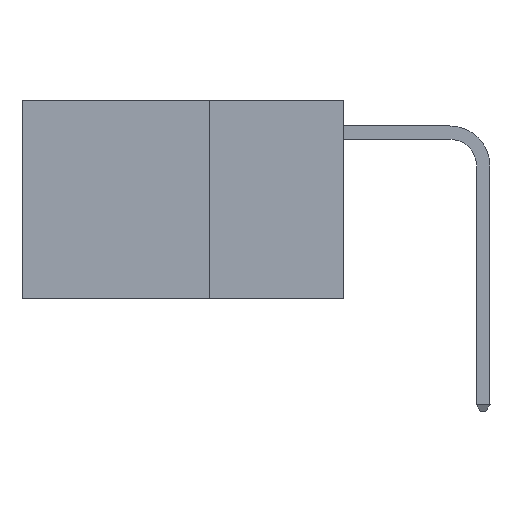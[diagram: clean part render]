
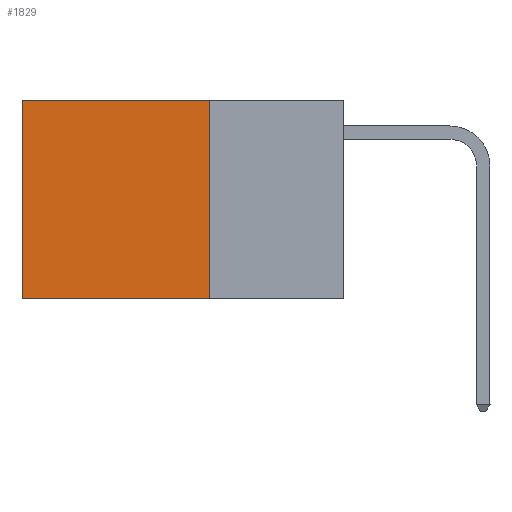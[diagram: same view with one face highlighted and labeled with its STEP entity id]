
A CAD part, left-side view. The second image highlights one B-rep face of the part: STEP entity #1829.
In plain terms, the highlighted planar face has unit normal (-1, 0, 0).
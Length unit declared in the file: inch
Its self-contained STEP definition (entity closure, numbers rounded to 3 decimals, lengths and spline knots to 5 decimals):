
#61 = EDGE_CURVE ( 'NONE', #5721, #1427, #5950, .T. ) ;
#127 = EDGE_CURVE ( 'NONE', #5721, #3329, #2680, .T. ) ;
#220 = PLANE ( 'NONE',  #3698 ) ;
#807 = CARTESIAN_POINT ( 'NONE',  ( 0.2625, 0.25, 0. ) ) ;
#833 = CARTESIAN_POINT ( 'NONE',  ( 0.2625, 0.25, 0. ) ) ;
#1358 = DIRECTION ( 'NONE',  ( 0., 0., -1. ) ) ;
#1413 = VECTOR ( 'NONE', #7861, 39.37008 ) ;
#1427 = VERTEX_POINT ( 'NONE', #7949 ) ;
#1829 = ADVANCED_FACE ( 'NONE', ( #3188 ), #220, .F. ) ;
#2013 = CARTESIAN_POINT ( 'NONE',  ( 0.2625, 0.25, -0.37 ) ) ;
#2420 = VECTOR ( 'NONE', #8285, 39.37008 ) ;
#2680 = LINE ( 'NONE', #5783, #2968 ) ;
#2968 = VECTOR ( 'NONE', #8905, 39.37008 ) ;
#3188 = FACE_OUTER_BOUND ( 'NONE', #7312, .T. ) ;
#3248 = DIRECTION ( 'NONE',  ( 1., 0., 0. ) ) ;
#3329 = VERTEX_POINT ( 'NONE', #4939 ) ;
#3698 = AXIS2_PLACEMENT_3D ( 'NONE', #807, #3248, #7219 ) ;
#3775 = EDGE_CURVE ( 'NONE', #1427, #8140, #5846, .T. ) ;
#4640 = CARTESIAN_POINT ( 'NONE',  ( 0.2625, 0.6, -0.37 ) ) ;
#4756 = VECTOR ( 'NONE', #1358, 39.37008 ) ;
#4757 = CARTESIAN_POINT ( 'NONE',  ( 0.2625, 0.6, 0. ) ) ;
#4939 = CARTESIAN_POINT ( 'NONE',  ( 0.2625, 0.6, 0. ) ) ;
#5721 = VERTEX_POINT ( 'NONE', #833 ) ;
#5783 = CARTESIAN_POINT ( 'NONE',  ( 0.2625, 0.25, 0. ) ) ;
#5846 = LINE ( 'NONE', #2013, #2420 ) ;
#5950 = LINE ( 'NONE', #9071, #4756 ) ;
#7047 = ORIENTED_EDGE ( 'NONE', *, *, #61, .F. ) ;
#7219 = DIRECTION ( 'NONE',  ( 0., 0., -1. ) ) ;
#7246 = ORIENTED_EDGE ( 'NONE', *, *, #3775, .F. ) ;
#7312 = EDGE_LOOP ( 'NONE', ( #7523, #7246, #7047, #9655 ) ) ;
#7523 = ORIENTED_EDGE ( 'NONE', *, *, #8175, .T. ) ;
#7861 = DIRECTION ( 'NONE',  ( 0., 0., -1. ) ) ;
#7949 = CARTESIAN_POINT ( 'NONE',  ( 0.2625, 0.25, -0.37 ) ) ;
#8140 = VERTEX_POINT ( 'NONE', #4640 ) ;
#8175 = EDGE_CURVE ( 'NONE', #3329, #8140, #8652, .T. ) ;
#8285 = DIRECTION ( 'NONE',  ( 0., 1., 0. ) ) ;
#8652 = LINE ( 'NONE', #4757, #1413 ) ;
#8905 = DIRECTION ( 'NONE',  ( 0., 1., 0. ) ) ;
#9071 = CARTESIAN_POINT ( 'NONE',  ( 0.2625, 0.25, 0. ) ) ;
#9655 = ORIENTED_EDGE ( 'NONE', *, *, #127, .T. ) ;
